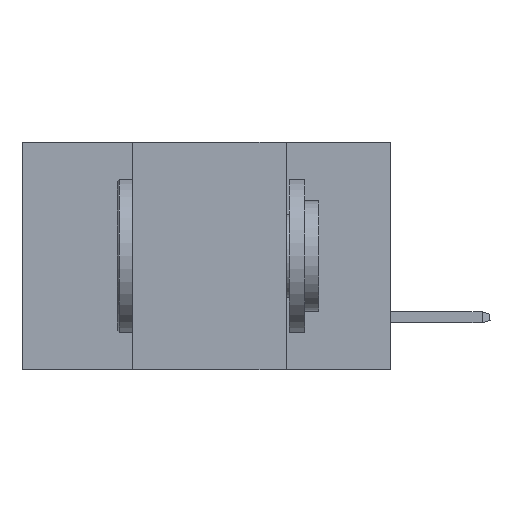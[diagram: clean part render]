
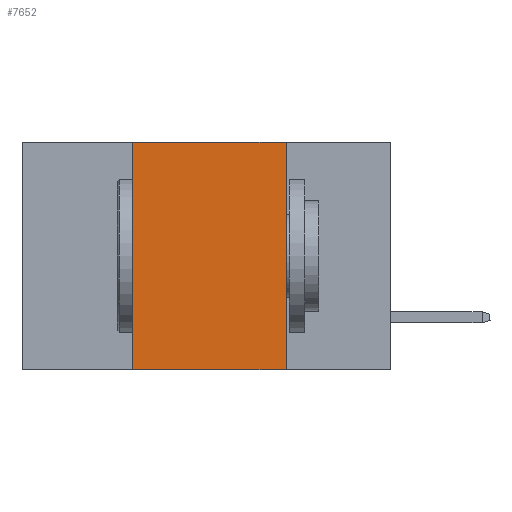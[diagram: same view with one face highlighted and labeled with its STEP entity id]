
A CAD part, left-side view. The second image highlights one B-rep face of the part: STEP entity #7652.
In plain terms, the highlighted planar face has unit normal (-1, 0, 0).
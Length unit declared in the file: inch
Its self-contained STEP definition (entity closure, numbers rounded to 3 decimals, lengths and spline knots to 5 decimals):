
#305 = VERTEX_POINT ( 'NONE', #10920 ) ;
#549 = VERTEX_POINT ( 'NONE', #8749 ) ;
#1772 = DIRECTION ( 'NONE',  ( 0., -1., 0. ) ) ;
#3207 = DIRECTION ( 'NONE',  ( 1., 0., 0. ) ) ;
#3964 = CARTESIAN_POINT ( 'NONE',  ( 0., 0.6, 0. ) ) ;
#4250 = CARTESIAN_POINT ( 'NONE',  ( 0., 0.17, 0. ) ) ;
#4277 = VERTEX_POINT ( 'NONE', #16269 ) ;
#4446 = PLANE ( 'NONE',  #6877 ) ;
#6877 = AXIS2_PLACEMENT_3D ( 'NONE', #14996, #3207, #26422 ) ;
#7652 = ADVANCED_FACE ( 'NONE', ( #16794 ), #4446, .F. ) ;
#8025 = VECTOR ( 'NONE', #1772, 39.37008 ) ;
#8540 = EDGE_CURVE ( 'NONE', #305, #20602, #8998, .T. ) ;
#8749 = CARTESIAN_POINT ( 'NONE',  ( 0., 0.42, -0.37 ) ) ;
#8843 = LINE ( 'NONE', #30697, #22714 ) ;
#8998 = LINE ( 'NONE', #4250, #15150 ) ;
#10784 = EDGE_CURVE ( 'NONE', #549, #20602, #33298, .T. ) ;
#10920 = CARTESIAN_POINT ( 'NONE',  ( 0., 0.17, 0. ) ) ;
#13719 = VECTOR ( 'NONE', #22554, 39.37008 ) ;
#14996 = CARTESIAN_POINT ( 'NONE',  ( 0., 0.6, 0. ) ) ;
#15150 = VECTOR ( 'NONE', #19927, 39.37008 ) ;
#15219 = ORIENTED_EDGE ( 'NONE', *, *, #16588, .F. ) ;
#15492 = ORIENTED_EDGE ( 'NONE', *, *, #10784, .T. ) ;
#16269 = CARTESIAN_POINT ( 'NONE',  ( 0., 0.42, 0. ) ) ;
#16588 = EDGE_CURVE ( 'NONE', #4277, #305, #20703, .T. ) ;
#16794 = FACE_OUTER_BOUND ( 'NONE', #27074, .T. ) ;
#16835 = ORIENTED_EDGE ( 'NONE', *, *, #25248, .F. ) ;
#17360 = CARTESIAN_POINT ( 'NONE',  ( 0., 0.6, -0.37 ) ) ;
#18513 = ORIENTED_EDGE ( 'NONE', *, *, #8540, .F. ) ;
#19927 = DIRECTION ( 'NONE',  ( 0., 0., -1. ) ) ;
#20602 = VERTEX_POINT ( 'NONE', #29093 ) ;
#20703 = LINE ( 'NONE', #3964, #13719 ) ;
#22554 = DIRECTION ( 'NONE',  ( 0., -1., 0. ) ) ;
#22714 = VECTOR ( 'NONE', #28228, 39.37008 ) ;
#25248 = EDGE_CURVE ( 'NONE', #549, #4277, #8843, .T. ) ;
#26422 = DIRECTION ( 'NONE',  ( 0., 0., -1. ) ) ;
#27074 = EDGE_LOOP ( 'NONE', ( #18513, #15219, #16835, #15492 ) ) ;
#28228 = DIRECTION ( 'NONE',  ( 0., 0., 1. ) ) ;
#29093 = CARTESIAN_POINT ( 'NONE',  ( 0., 0.17, -0.37 ) ) ;
#30697 = CARTESIAN_POINT ( 'NONE',  ( 0., 0.42, 0. ) ) ;
#33298 = LINE ( 'NONE', #17360, #8025 ) ;
